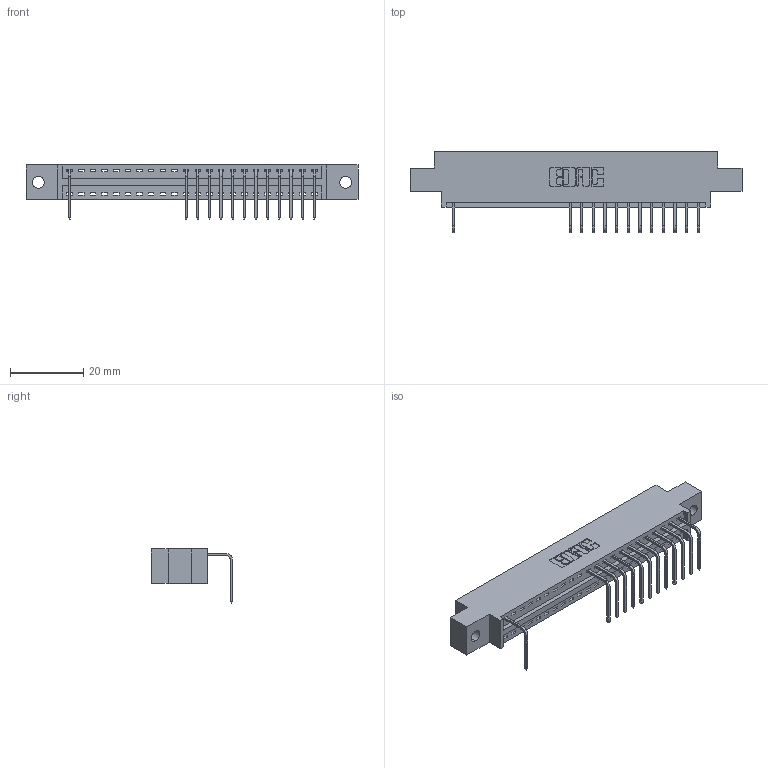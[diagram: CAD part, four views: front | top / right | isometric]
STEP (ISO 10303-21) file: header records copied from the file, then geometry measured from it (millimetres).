
FILE_DESCRIPTION (( 'STEP AP203' ), '1' );
FILE_NAME ('346-022-558-602.STEP', '2018-08-21T01:08:05', ( '' ), ( '' ), 'SwSTEP 2.0', 'SolidWorks 2016', '' );
FILE_SCHEMA (( 'CONFIG_CONTROL_DESIGN' ));
Length unit declared in the file: inch
Products named in the file (3): 346 Part_0.170 Offset - 0.128 Dia; 345-292-001_558 Tail - 2; 346-022-558-602
Assembly tree (14 placements, depth 2):
  346-022-558-602
    346 Part_0.170 Offset - 0.128 Dia
    345-292-001_558 Tail - 2  x13
Bounding box: 90.42 x 22.16 x 14.73 mm (x, y, z)
Volume: 8266.9 mm3; surface area: 9710.4 mm2
Topology: 14 solids, 14 shells, 1014 faces, 3085 edges, 2038 vertices
Faces by surface type: plane 716, cylinder 298
Entity records: 16277 total; most frequent: CARTESIAN_POINT 2845, ORIENTED_EDGE 2810, DIRECTION 2523, EDGE_CURVE 1405, LINE 1185, VECTOR 1185, VERTEX_POINT 934, AXIS2_PLACEMENT_3D 669
